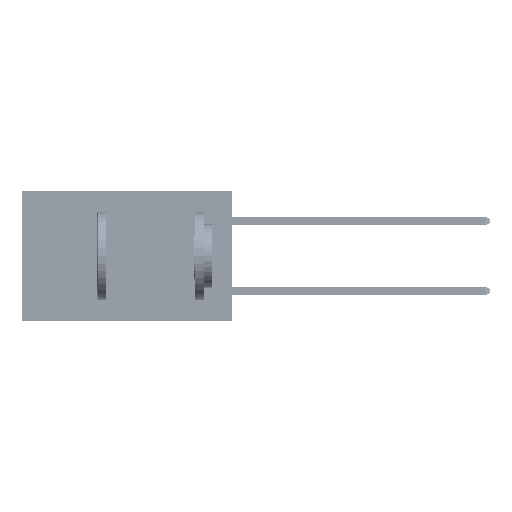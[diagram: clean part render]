
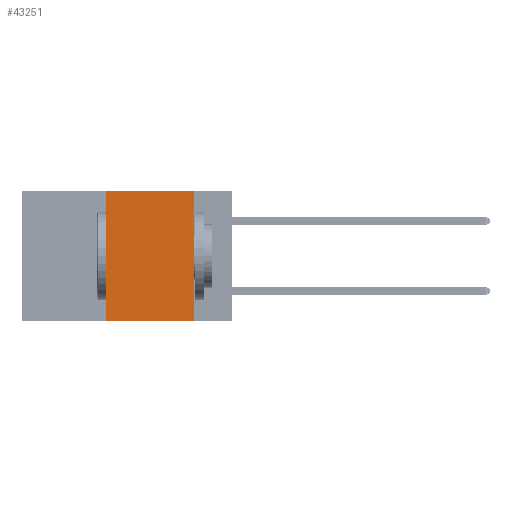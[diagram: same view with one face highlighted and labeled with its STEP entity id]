
A CAD part, left-side view. The second image highlights one B-rep face of the part: STEP entity #43251.
In plain terms, the highlighted planar face has unit normal (-1, 0, 0).
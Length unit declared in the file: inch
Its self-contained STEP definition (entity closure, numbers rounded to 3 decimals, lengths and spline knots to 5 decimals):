
#250 = VERTEX_POINT ( 'NONE', #476 ) ;
#339 = ORIENTED_EDGE ( 'NONE', *, *, #8040, .F. ) ;
#476 = CARTESIAN_POINT ( 'NONE',  ( 0., 0.11, 0. ) ) ;
#2582 = CARTESIAN_POINT ( 'NONE',  ( 0., 0.11, 0. ) ) ;
#6328 = VECTOR ( 'NONE', #40567, 39.37008 ) ;
#6445 = FACE_OUTER_BOUND ( 'NONE', #31174, .T. ) ;
#6780 = ORIENTED_EDGE ( 'NONE', *, *, #36578, .F. ) ;
#8040 = EDGE_CURVE ( 'NONE', #250, #12265, #20251, .T. ) ;
#8109 = EDGE_CURVE ( 'NONE', #15259, #12265, #41580, .T. ) ;
#9832 = CARTESIAN_POINT ( 'NONE',  ( 0., 0.11, -0.37 ) ) ;
#10297 = CARTESIAN_POINT ( 'NONE',  ( 0., 0.36, -0.37 ) ) ;
#12265 = VERTEX_POINT ( 'NONE', #9832 ) ;
#12906 = EDGE_CURVE ( 'NONE', #15259, #14157, #36594, .T. ) ;
#13204 = VECTOR ( 'NONE', #19085, 39.37008 ) ;
#13943 = CARTESIAN_POINT ( 'NONE',  ( 0., 0.6, 0. ) ) ;
#14157 = VERTEX_POINT ( 'NONE', #26122 ) ;
#15208 = CARTESIAN_POINT ( 'NONE',  ( 0., 0.6, -0.37 ) ) ;
#15259 = VERTEX_POINT ( 'NONE', #10297 ) ;
#17964 = LINE ( 'NONE', #26587, #13204 ) ;
#18068 = CARTESIAN_POINT ( 'NONE',  ( 0., 0.36, 0. ) ) ;
#19085 = DIRECTION ( 'NONE',  ( 0., -1., 0. ) ) ;
#20112 = AXIS2_PLACEMENT_3D ( 'NONE', #13943, #40604, #33146 ) ;
#20251 = LINE ( 'NONE', #2582, #47531 ) ;
#26122 = CARTESIAN_POINT ( 'NONE',  ( 0., 0.36, 0. ) ) ;
#26587 = CARTESIAN_POINT ( 'NONE',  ( 0., 0.6, 0. ) ) ;
#29016 = PLANE ( 'NONE',  #20112 ) ;
#29638 = DIRECTION ( 'NONE',  ( 0., 0., -1. ) ) ;
#30455 = ORIENTED_EDGE ( 'NONE', *, *, #8109, .T. ) ;
#31174 = EDGE_LOOP ( 'NONE', ( #339, #6780, #38613, #30455 ) ) ;
#32688 = VECTOR ( 'NONE', #34090, 39.37008 ) ;
#33146 = DIRECTION ( 'NONE',  ( 0., 0., -1. ) ) ;
#34090 = DIRECTION ( 'NONE',  ( 0., -1., 0. ) ) ;
#36578 = EDGE_CURVE ( 'NONE', #14157, #250, #17964, .T. ) ;
#36594 = LINE ( 'NONE', #18068, #6328 ) ;
#38613 = ORIENTED_EDGE ( 'NONE', *, *, #12906, .F. ) ;
#40567 = DIRECTION ( 'NONE',  ( 0., 0., 1. ) ) ;
#40604 = DIRECTION ( 'NONE',  ( 1., 0., 0. ) ) ;
#41580 = LINE ( 'NONE', #15208, #32688 ) ;
#43251 = ADVANCED_FACE ( 'NONE', ( #6445 ), #29016, .F. ) ;
#47531 = VECTOR ( 'NONE', #29638, 39.37008 ) ;
